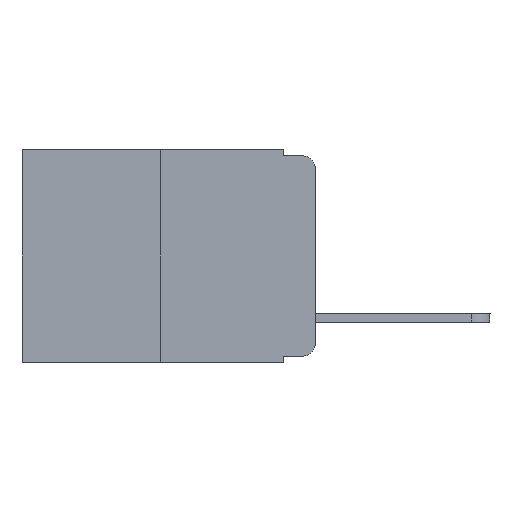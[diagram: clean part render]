
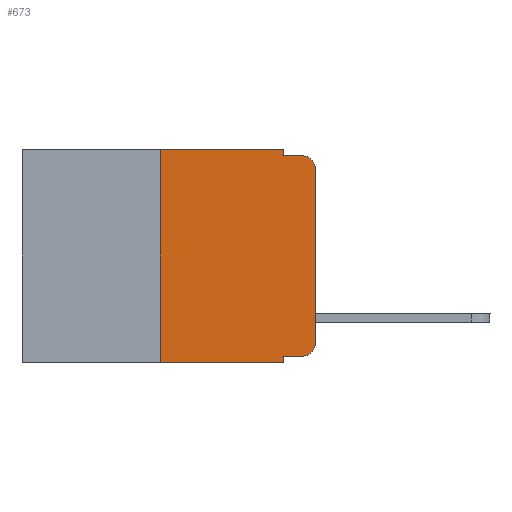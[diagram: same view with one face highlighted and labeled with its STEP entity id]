
A CAD part, left-side view. The second image highlights one B-rep face of the part: STEP entity #673.
In plain terms, the highlighted planar face has unit normal (-1, 0, 0).
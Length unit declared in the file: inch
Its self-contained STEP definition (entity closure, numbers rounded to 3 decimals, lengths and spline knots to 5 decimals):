
#14 = LINE ( 'NONE', #8065, #7727 ) ;
#39 = EDGE_CURVE ( 'NONE', #7841, #7319, #3536, .T. ) ;
#86 = CARTESIAN_POINT ( 'NONE',  ( 0., 0.051, -0.343 ) ) ;
#621 = CARTESIAN_POINT ( 'NONE',  ( 0., 0.051, 0. ) ) ;
#673 = ADVANCED_FACE ( 'NONE', ( #4785 ), #19456, .F. ) ;
#814 = LINE ( 'NONE', #17059, #9051 ) ;
#1228 = EDGE_CURVE ( 'NONE', #10574, #15198, #10924, .T. ) ;
#1421 = EDGE_CURVE ( 'NONE', #1761, #15198, #8829, .T. ) ;
#1576 = DIRECTION ( 'NONE',  ( 0., -1., 0. ) ) ;
#1761 = VERTEX_POINT ( 'NONE', #2213 ) ;
#1800 = LINE ( 'NONE', #5884, #9509 ) ;
#1898 = LINE ( 'NONE', #3576, #9882 ) ;
#1979 = CARTESIAN_POINT ( 'NONE',  ( 0., 0.02, -0.03 ) ) ;
#2213 = CARTESIAN_POINT ( 'NONE',  ( 0., 0.25, -0.343 ) ) ;
#2366 = ORIENTED_EDGE ( 'NONE', *, *, #4420, .T. ) ;
#2367 = ORIENTED_EDGE ( 'NONE', *, *, #20784, .T. ) ;
#2628 = VERTEX_POINT ( 'NONE', #4308 ) ;
#3150 = AXIS2_PLACEMENT_3D ( 'NONE', #7250, #16976, #7102 ) ;
#3430 = DIRECTION ( 'NONE',  ( 0., 0., -1. ) ) ;
#3536 = LINE ( 'NONE', #19692, #11746 ) ;
#3576 = CARTESIAN_POINT ( 'NONE',  ( 0., 0., 0. ) ) ;
#3784 = EDGE_CURVE ( 'NONE', #7319, #13313, #10525, .T. ) ;
#4308 = CARTESIAN_POINT ( 'NONE',  ( 0., 0., -0.03 ) ) ;
#4420 = EDGE_CURVE ( 'NONE', #10574, #20182, #1800, .T. ) ;
#4477 = VECTOR ( 'NONE', #10983, 39.37008 ) ;
#4785 = FACE_OUTER_BOUND ( 'NONE', #13914, .T. ) ;
#5103 = EDGE_CURVE ( 'NONE', #20182, #15339, #18458, .T. ) ;
#5884 = CARTESIAN_POINT ( 'NONE',  ( 0., 0.051, -0.333 ) ) ;
#6015 = CARTESIAN_POINT ( 'NONE',  ( 0., 0.473, -0.343 ) ) ;
#6418 = DIRECTION ( 'NONE',  ( 0., 0., -1. ) ) ;
#6482 = CARTESIAN_POINT ( 'NONE',  ( 0., 0.051, 0. ) ) ;
#6834 = DIRECTION ( 'NONE',  ( -1., 0., 0. ) ) ;
#7102 = DIRECTION ( 'NONE',  ( 0., 0., -1. ) ) ;
#7250 = CARTESIAN_POINT ( 'NONE',  ( 0., 0.02, -0.313 ) ) ;
#7319 = VERTEX_POINT ( 'NONE', #8059 ) ;
#7727 = VECTOR ( 'NONE', #11073, 39.37008 ) ;
#7841 = VERTEX_POINT ( 'NONE', #14585 ) ;
#8059 = CARTESIAN_POINT ( 'NONE',  ( 0., 0.051, 0. ) ) ;
#8065 = CARTESIAN_POINT ( 'NONE',  ( 0., 0.051, -0.01 ) ) ;
#8173 = AXIS2_PLACEMENT_3D ( 'NONE', #1979, #6834, #8444 ) ;
#8302 = ORIENTED_EDGE ( 'NONE', *, *, #13021, .F. ) ;
#8444 = DIRECTION ( 'NONE',  ( 0., 0., -1. ) ) ;
#8633 = ORIENTED_EDGE ( 'NONE', *, *, #3784, .F. ) ;
#8829 = LINE ( 'NONE', #6015, #4477 ) ;
#9051 = VECTOR ( 'NONE', #11960, 39.37008 ) ;
#9147 = VERTEX_POINT ( 'NONE', #14690 ) ;
#9159 = CARTESIAN_POINT ( 'NONE',  ( 0., 0.051, -0.333 ) ) ;
#9509 = VECTOR ( 'NONE', #13994, 39.37008 ) ;
#9817 = CARTESIAN_POINT ( 'NONE',  ( 0., 0.473, 0. ) ) ;
#9882 = VECTOR ( 'NONE', #13208, 39.37008 ) ;
#10140 = CARTESIAN_POINT ( 'NONE',  ( 0., 0.02, -0.333 ) ) ;
#10419 = ORIENTED_EDGE ( 'NONE', *, *, #18100, .T. ) ;
#10525 = LINE ( 'NONE', #6482, #10799 ) ;
#10574 = VERTEX_POINT ( 'NONE', #9159 ) ;
#10799 = VECTOR ( 'NONE', #3430, 39.37008 ) ;
#10924 = LINE ( 'NONE', #621, #19926 ) ;
#10983 = DIRECTION ( 'NONE',  ( 0., -1., 0. ) ) ;
#11073 = DIRECTION ( 'NONE',  ( 0., -1., 0. ) ) ;
#11746 = VECTOR ( 'NONE', #1576, 39.37008 ) ;
#11879 = ORIENTED_EDGE ( 'NONE', *, *, #1228, .F. ) ;
#11941 = CARTESIAN_POINT ( 'NONE',  ( 0., 0., -0.313 ) ) ;
#11960 = DIRECTION ( 'NONE',  ( 0., 0., 1. ) ) ;
#12294 = DIRECTION ( 'NONE',  ( 0., 0., -1. ) ) ;
#12890 = CARTESIAN_POINT ( 'NONE',  ( 0., 0.051, -0.01 ) ) ;
#13021 = EDGE_CURVE ( 'NONE', #1761, #7841, #814, .T. ) ;
#13208 = DIRECTION ( 'NONE',  ( 0., 0., 1. ) ) ;
#13313 = VERTEX_POINT ( 'NONE', #12890 ) ;
#13711 = EDGE_CURVE ( 'NONE', #13313, #9147, #14, .T. ) ;
#13914 = EDGE_LOOP ( 'NONE', ( #10419, #2367, #15041, #8633, #17001, #8302, #14619, #11879, #2366, #16669 ) ) ;
#13994 = DIRECTION ( 'NONE',  ( 0., -1., 0. ) ) ;
#14585 = CARTESIAN_POINT ( 'NONE',  ( 0., 0.25, 0. ) ) ;
#14619 = ORIENTED_EDGE ( 'NONE', *, *, #1421, .T. ) ;
#14690 = CARTESIAN_POINT ( 'NONE',  ( 0., 0.02, -0.01 ) ) ;
#14879 = AXIS2_PLACEMENT_3D ( 'NONE', #9817, #17871, #6418 ) ;
#15041 = ORIENTED_EDGE ( 'NONE', *, *, #13711, .F. ) ;
#15198 = VERTEX_POINT ( 'NONE', #86 ) ;
#15339 = VERTEX_POINT ( 'NONE', #11941 ) ;
#16669 = ORIENTED_EDGE ( 'NONE', *, *, #5103, .T. ) ;
#16976 = DIRECTION ( 'NONE',  ( -1., 0., 0. ) ) ;
#17001 = ORIENTED_EDGE ( 'NONE', *, *, #39, .F. ) ;
#17059 = CARTESIAN_POINT ( 'NONE',  ( 0., 0.25, 0. ) ) ;
#17622 = CIRCLE ( 'NONE', #8173, 0.02 ) ;
#17871 = DIRECTION ( 'NONE',  ( 1., 0., 0. ) ) ;
#18100 = EDGE_CURVE ( 'NONE', #15339, #2628, #1898, .T. ) ;
#18458 = CIRCLE ( 'NONE', #3150, 0.02 ) ;
#19456 = PLANE ( 'NONE',  #14879 ) ;
#19692 = CARTESIAN_POINT ( 'NONE',  ( 0., 0.473, 0. ) ) ;
#19926 = VECTOR ( 'NONE', #12294, 39.37008 ) ;
#20182 = VERTEX_POINT ( 'NONE', #10140 ) ;
#20784 = EDGE_CURVE ( 'NONE', #2628, #9147, #17622, .T. ) ;
